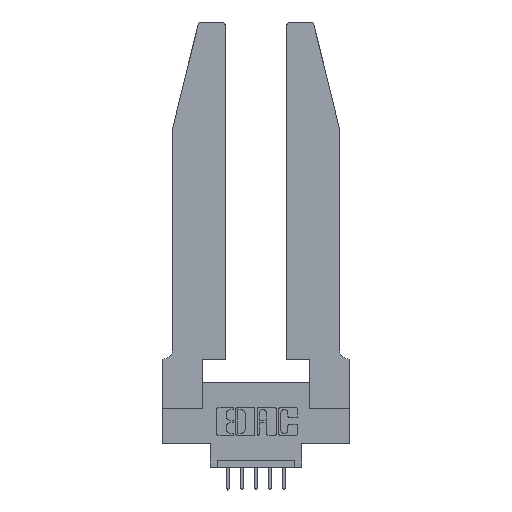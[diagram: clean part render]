
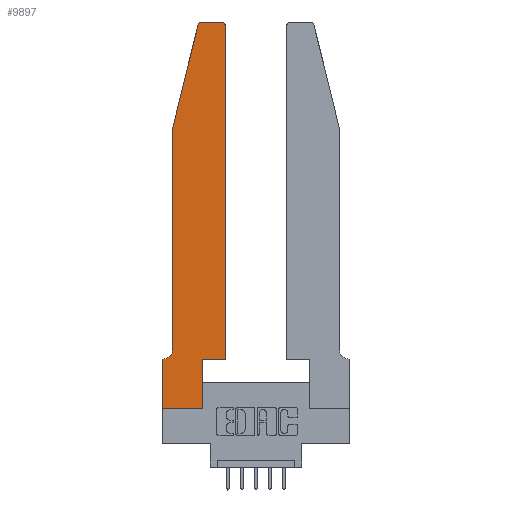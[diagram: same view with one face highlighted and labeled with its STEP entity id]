
A CAD part, top view. The second image highlights one B-rep face of the part: STEP entity #9897.
In plain terms, the highlighted planar face has unit normal (0, 0, 1).
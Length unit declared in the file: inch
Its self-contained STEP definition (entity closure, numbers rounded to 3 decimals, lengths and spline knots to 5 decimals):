
#88 = ORIENTED_EDGE ( 'NONE', *, *, #9273, .T. ) ;
#104 = CARTESIAN_POINT ( 'NONE',  ( 0., 0.35, 0.37 ) ) ;
#258 = DIRECTION ( 'NONE',  ( 0., 0., 1. ) ) ;
#460 = VECTOR ( 'NONE', #10780, 39.37008 ) ;
#476 = DIRECTION ( 'NONE',  ( 0., 0., -1. ) ) ;
#551 = EDGE_CURVE ( 'NONE', #11446, #5759, #1509, .T. ) ;
#790 = CARTESIAN_POINT ( 'NONE',  ( 0., 0., 0.37 ) ) ;
#812 = DIRECTION ( 'NONE',  ( 1., 0., 0. ) ) ;
#829 = DIRECTION ( 'NONE',  ( 1., 0., 0. ) ) ;
#880 = ORIENTED_EDGE ( 'NONE', *, *, #5864, .T. ) ;
#988 = VECTOR ( 'NONE', #11467, 39.37008 ) ;
#1109 = VERTEX_POINT ( 'NONE', #8237 ) ;
#1167 = PLANE ( 'NONE',  #4625 ) ;
#1253 = EDGE_CURVE ( 'NONE', #10375, #11446, #9414, .T. ) ;
#1509 = LINE ( 'NONE', #9094, #8780 ) ;
#1539 = DIRECTION ( 'NONE',  ( 0., -1., 0. ) ) ;
#1710 = CARTESIAN_POINT ( 'NONE',  ( 0.0755, 0.42, 0.37 ) ) ;
#1767 = DIRECTION ( 'NONE',  ( 0., -1., 0. ) ) ;
#1830 = LINE ( 'NONE', #5096, #2999 ) ;
#1925 = VERTEX_POINT ( 'NONE', #11694 ) ;
#2483 = EDGE_CURVE ( 'NONE', #8575, #1925, #6089, .T. ) ;
#2543 = CARTESIAN_POINT ( 'NONE',  ( 0.0055, 0.35, 0.37 ) ) ;
#2836 = LINE ( 'NONE', #5950, #9579 ) ;
#2864 = CARTESIAN_POINT ( 'NONE',  ( 0.4205, 2.72, 0.37 ) ) ;
#2999 = VECTOR ( 'NONE', #13410, 39.37008 ) ;
#3139 = ORIENTED_EDGE ( 'NONE', *, *, #6669, .T. ) ;
#3267 = LINE ( 'NONE', #10535, #12497 ) ;
#3658 = AXIS2_PLACEMENT_3D ( 'NONE', #2864, #7122, #812 ) ;
#4407 = VERTEX_POINT ( 'NONE', #7721 ) ;
#4625 = AXIS2_PLACEMENT_3D ( 'NONE', #104, #12815, #11683 ) ;
#4647 = AXIS2_PLACEMENT_3D ( 'NONE', #12075, #258, #10891 ) ;
#4736 = ORIENTED_EDGE ( 'NONE', *, *, #7674, .T. ) ;
#4947 = VERTEX_POINT ( 'NONE', #6758 ) ;
#5096 = CARTESIAN_POINT ( 'NONE',  ( 0.2865, 0.35, 0.37 ) ) ;
#5149 = EDGE_CURVE ( 'NONE', #1925, #9464, #8493, .T. ) ;
#5302 = CIRCLE ( 'NONE', #4647, 0.03 ) ;
#5759 = VERTEX_POINT ( 'NONE', #7576 ) ;
#5864 = EDGE_CURVE ( 'NONE', #5759, #7325, #11100, .T. ) ;
#5950 = CARTESIAN_POINT ( 'NONE',  ( 0.0755, 2., 0.37 ) ) ;
#6024 = ORIENTED_EDGE ( 'NONE', *, *, #7715, .T. ) ;
#6039 = ORIENTED_EDGE ( 'NONE', *, *, #551, .T. ) ;
#6089 = LINE ( 'NONE', #8364, #460 ) ;
#6143 = VERTEX_POINT ( 'NONE', #8784 ) ;
#6656 = CARTESIAN_POINT ( 'NONE',  ( 0., 0., 0.37 ) ) ;
#6669 = EDGE_CURVE ( 'NONE', #9464, #4407, #11914, .T. ) ;
#6758 = CARTESIAN_POINT ( 'NONE',  ( 0.2865, 0.35, 0.37 ) ) ;
#6800 = CARTESIAN_POINT ( 'NONE',  ( 0.0055, 0.42, 0.37 ) ) ;
#6829 = DIRECTION ( 'NONE',  ( -1., 0., 0. ) ) ;
#7012 = EDGE_CURVE ( 'NONE', #4407, #1109, #5302, .T. ) ;
#7122 = DIRECTION ( 'NONE',  ( 0., 0., 1. ) ) ;
#7325 = VERTEX_POINT ( 'NONE', #13203 ) ;
#7576 = CARTESIAN_POINT ( 'NONE',  ( 0., 0.35, 0.37 ) ) ;
#7674 = EDGE_CURVE ( 'NONE', #10675, #4947, #1830, .T. ) ;
#7715 = EDGE_CURVE ( 'NONE', #6143, #10375, #2836, .T. ) ;
#7721 = CARTESIAN_POINT ( 'NONE',  ( 0.284, 2.75, 0.37 ) ) ;
#8028 = AXIS2_PLACEMENT_3D ( 'NONE', #6800, #476, #9978 ) ;
#8161 = LINE ( 'NONE', #790, #9330 ) ;
#8237 = CARTESIAN_POINT ( 'NONE',  ( 0.25487, 2.72718, 0.37 ) ) ;
#8350 = DIRECTION ( 'NONE',  ( 1., 0., 0. ) ) ;
#8364 = CARTESIAN_POINT ( 'NONE',  ( 0.4505, 0.35, 0.37 ) ) ;
#8493 = CIRCLE ( 'NONE', #3658, 0.03 ) ;
#8575 = VERTEX_POINT ( 'NONE', #10047 ) ;
#8780 = VECTOR ( 'NONE', #6829, 39.37008 ) ;
#8784 = CARTESIAN_POINT ( 'NONE',  ( 0.0755, 2., 0.37 ) ) ;
#9094 = CARTESIAN_POINT ( 'NONE',  ( 0.0755, 0.35, 0.37 ) ) ;
#9273 = EDGE_CURVE ( 'NONE', #1109, #6143, #9569, .T. ) ;
#9303 = VECTOR ( 'NONE', #1539, 39.37008 ) ;
#9330 = VECTOR ( 'NONE', #829, 39.37008 ) ;
#9414 = CIRCLE ( 'NONE', #8028, 0.07 ) ;
#9464 = VERTEX_POINT ( 'NONE', #12916 ) ;
#9503 = ORIENTED_EDGE ( 'NONE', *, *, #11140, .T. ) ;
#9569 = LINE ( 'NONE', #11656, #988 ) ;
#9579 = VECTOR ( 'NONE', #1767, 39.37008 ) ;
#9897 = ADVANCED_FACE ( 'NONE', ( #13213 ), #1167, .T. ) ;
#9978 = DIRECTION ( 'NONE',  ( -1., 0., 0. ) ) ;
#10047 = CARTESIAN_POINT ( 'NONE',  ( 0.4505, 0.35, 0.37 ) ) ;
#10094 = ORIENTED_EDGE ( 'NONE', *, *, #7012, .T. ) ;
#10375 = VERTEX_POINT ( 'NONE', #1710 ) ;
#10535 = CARTESIAN_POINT ( 'NONE',  ( 0.4505, 0.35, 0.37 ) ) ;
#10675 = VERTEX_POINT ( 'NONE', #11007 ) ;
#10748 = VECTOR ( 'NONE', #13387, 39.37008 ) ;
#10780 = DIRECTION ( 'NONE',  ( 0., 1., 0. ) ) ;
#10891 = DIRECTION ( 'NONE',  ( 1., 0., 0. ) ) ;
#11007 = CARTESIAN_POINT ( 'NONE',  ( 0.2865, 0., 0.37 ) ) ;
#11100 = LINE ( 'NONE', #6656, #9303 ) ;
#11140 = EDGE_CURVE ( 'NONE', #4947, #8575, #3267, .T. ) ;
#11446 = VERTEX_POINT ( 'NONE', #2543 ) ;
#11467 = DIRECTION ( 'NONE',  ( -0.239, -0.971, 0. ) ) ;
#11656 = CARTESIAN_POINT ( 'NONE',  ( 0.0755, 2., 0.37 ) ) ;
#11683 = DIRECTION ( 'NONE',  ( 1., 0., 0. ) ) ;
#11694 = CARTESIAN_POINT ( 'NONE',  ( 0.4505, 2.72, 0.37 ) ) ;
#11914 = LINE ( 'NONE', #13487, #10748 ) ;
#12075 = CARTESIAN_POINT ( 'NONE',  ( 0.284, 2.72, 0.37 ) ) ;
#12203 = EDGE_CURVE ( 'NONE', #7325, #10675, #8161, .T. ) ;
#12497 = VECTOR ( 'NONE', #8350, 39.37008 ) ;
#12589 = ORIENTED_EDGE ( 'NONE', *, *, #12203, .T. ) ;
#12617 = ORIENTED_EDGE ( 'NONE', *, *, #1253, .T. ) ;
#12815 = DIRECTION ( 'NONE',  ( 0., 0., 1. ) ) ;
#12834 = ORIENTED_EDGE ( 'NONE', *, *, #2483, .T. ) ;
#12881 = EDGE_LOOP ( 'NONE', ( #3139, #10094, #88, #6024, #12617, #6039, #880, #12589, #4736, #9503, #12834, #13095 ) ) ;
#12916 = CARTESIAN_POINT ( 'NONE',  ( 0.4205, 2.75, 0.37 ) ) ;
#13095 = ORIENTED_EDGE ( 'NONE', *, *, #5149, .T. ) ;
#13203 = CARTESIAN_POINT ( 'NONE',  ( 0., 0., 0.37 ) ) ;
#13213 = FACE_OUTER_BOUND ( 'NONE', #12881, .T. ) ;
#13387 = DIRECTION ( 'NONE',  ( -1., 0., 0. ) ) ;
#13410 = DIRECTION ( 'NONE',  ( 0., 1., 0. ) ) ;
#13487 = CARTESIAN_POINT ( 'NONE',  ( 0.2605, 2.75, 0.37 ) ) ;
